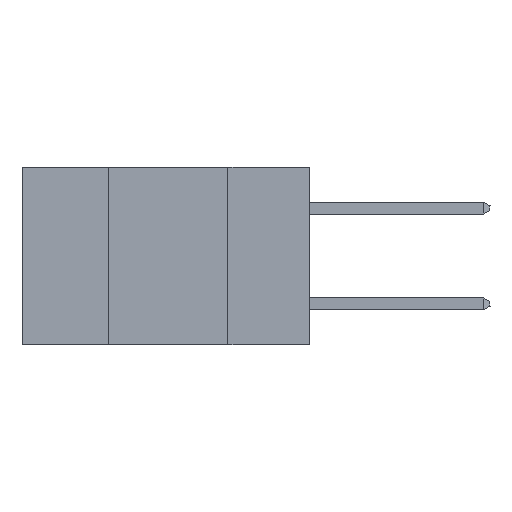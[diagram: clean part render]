
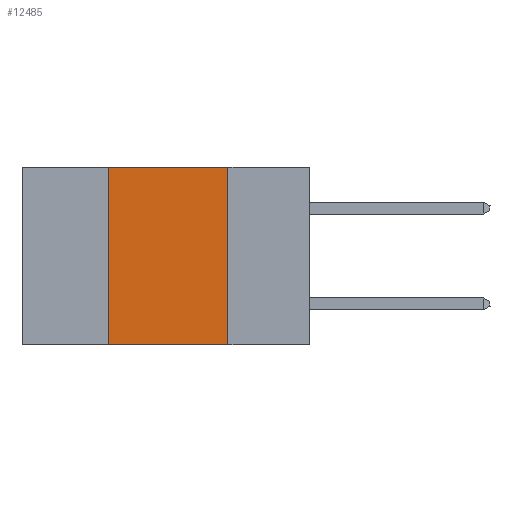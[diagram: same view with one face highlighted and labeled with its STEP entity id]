
A CAD part, left-side view. The second image highlights one B-rep face of the part: STEP entity #12485.
In plain terms, the highlighted planar face has unit normal (-1, 0, 0).
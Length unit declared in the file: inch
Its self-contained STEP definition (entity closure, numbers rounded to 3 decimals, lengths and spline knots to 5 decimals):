
#499 = VECTOR ( 'NONE', #13442, 39.37008 ) ;
#536 = CARTESIAN_POINT ( 'NONE',  ( 0., 0.17, 0. ) ) ;
#916 = EDGE_LOOP ( 'NONE', ( #12431, #11429, #9773, #8293 ) ) ;
#1023 = VECTOR ( 'NONE', #2803, 39.37008 ) ;
#1854 = EDGE_CURVE ( 'NONE', #7734, #6129, #4937, .T. ) ;
#1945 = VERTEX_POINT ( 'NONE', #4364 ) ;
#2803 = DIRECTION ( 'NONE',  ( 0., 0., -1. ) ) ;
#2993 = DIRECTION ( 'NONE',  ( 0., -1., 0. ) ) ;
#3158 = CARTESIAN_POINT ( 'NONE',  ( 0., 0.6, 0. ) ) ;
#3734 = FACE_OUTER_BOUND ( 'NONE', #916, .T. ) ;
#3954 = CARTESIAN_POINT ( 'NONE',  ( 0., 0.42, 0. ) ) ;
#4364 = CARTESIAN_POINT ( 'NONE',  ( 0., 0.17, 0. ) ) ;
#4937 = LINE ( 'NONE', #9082, #499 ) ;
#4996 = EDGE_CURVE ( 'NONE', #7734, #10657, #11124, .T. ) ;
#5439 = DIRECTION ( 'NONE',  ( 1., 0., 0. ) ) ;
#6129 = VERTEX_POINT ( 'NONE', #3954 ) ;
#6249 = VECTOR ( 'NONE', #2993, 39.37008 ) ;
#7310 = VECTOR ( 'NONE', #13703, 39.37008 ) ;
#7734 = VERTEX_POINT ( 'NONE', #10215 ) ;
#7993 = LINE ( 'NONE', #536, #1023 ) ;
#8293 = ORIENTED_EDGE ( 'NONE', *, *, #4996, .T. ) ;
#8806 = AXIS2_PLACEMENT_3D ( 'NONE', #3158, #5439, #12393 ) ;
#9082 = CARTESIAN_POINT ( 'NONE',  ( 0., 0.42, 0. ) ) ;
#9773 = ORIENTED_EDGE ( 'NONE', *, *, #1854, .F. ) ;
#9854 = CARTESIAN_POINT ( 'NONE',  ( 0., 0.6, -0.37 ) ) ;
#10013 = PLANE ( 'NONE',  #8806 ) ;
#10215 = CARTESIAN_POINT ( 'NONE',  ( 0., 0.42, -0.37 ) ) ;
#10657 = VERTEX_POINT ( 'NONE', #11968 ) ;
#11124 = LINE ( 'NONE', #9854, #6249 ) ;
#11336 = EDGE_CURVE ( 'NONE', #1945, #10657, #7993, .T. ) ;
#11429 = ORIENTED_EDGE ( 'NONE', *, *, #12561, .F. ) ;
#11968 = CARTESIAN_POINT ( 'NONE',  ( 0., 0.17, -0.37 ) ) ;
#12393 = DIRECTION ( 'NONE',  ( 0., 0., -1. ) ) ;
#12431 = ORIENTED_EDGE ( 'NONE', *, *, #11336, .F. ) ;
#12485 = ADVANCED_FACE ( 'NONE', ( #3734 ), #10013, .F. ) ;
#12561 = EDGE_CURVE ( 'NONE', #6129, #1945, #14138, .T. ) ;
#12695 = CARTESIAN_POINT ( 'NONE',  ( 0., 0.6, 0. ) ) ;
#13442 = DIRECTION ( 'NONE',  ( 0., 0., 1. ) ) ;
#13703 = DIRECTION ( 'NONE',  ( 0., -1., 0. ) ) ;
#14138 = LINE ( 'NONE', #12695, #7310 ) ;
